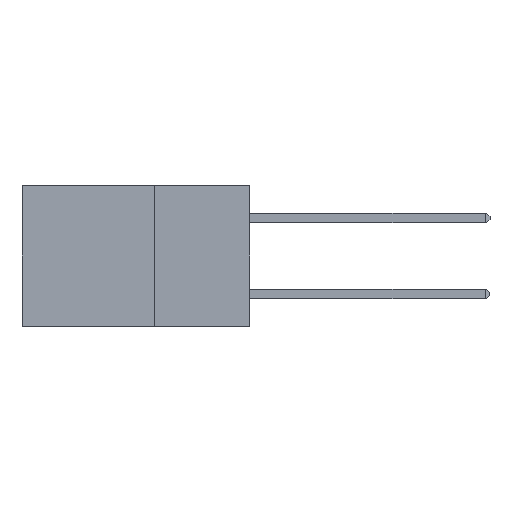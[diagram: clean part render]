
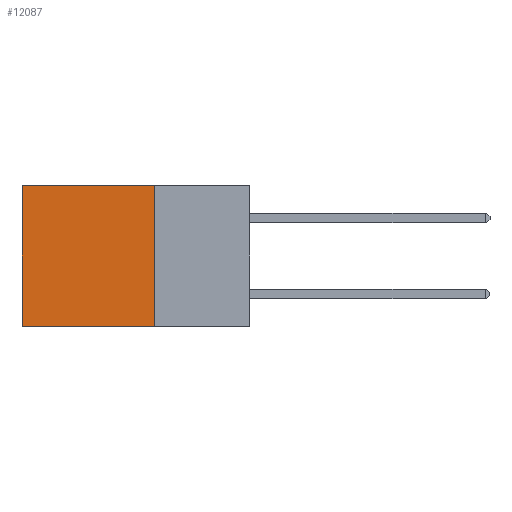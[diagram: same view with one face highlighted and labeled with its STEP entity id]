
A CAD part, left-side view. The second image highlights one B-rep face of the part: STEP entity #12087.
In plain terms, the highlighted planar face has unit normal (-1, 0, 0).
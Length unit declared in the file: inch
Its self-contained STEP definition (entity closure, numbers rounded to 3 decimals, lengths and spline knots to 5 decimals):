
#23 = CARTESIAN_POINT ( 'NONE',  ( 0.2875, 0.25, 0. ) ) ;
#40 = VECTOR ( 'NONE', #2135, 39.37008 ) ;
#397 = VECTOR ( 'NONE', #10074, 39.37008 ) ;
#904 = FACE_OUTER_BOUND ( 'NONE', #2620, .T. ) ;
#1497 = EDGE_CURVE ( 'NONE', #9863, #4979, #12409, .T. ) ;
#2125 = VERTEX_POINT ( 'NONE', #10823 ) ;
#2135 = DIRECTION ( 'NONE',  ( 0., 1., 0. ) ) ;
#2505 = CARTESIAN_POINT ( 'NONE',  ( 0.2875, 0.25, 0. ) ) ;
#2620 = EDGE_LOOP ( 'NONE', ( #8207, #11668, #6762, #9559 ) ) ;
#3856 = LINE ( 'NONE', #2505, #397 ) ;
#4747 = CARTESIAN_POINT ( 'NONE',  ( 0.2875, 0.25, 0. ) ) ;
#4979 = VERTEX_POINT ( 'NONE', #10751 ) ;
#5901 = CARTESIAN_POINT ( 'NONE',  ( 0.2875, 0.25, 0. ) ) ;
#6376 = EDGE_CURVE ( 'NONE', #4979, #8288, #9129, .T. ) ;
#6461 = DIRECTION ( 'NONE',  ( 0., 0., -1. ) ) ;
#6762 = ORIENTED_EDGE ( 'NONE', *, *, #15653, .F. ) ;
#7368 = CARTESIAN_POINT ( 'NONE',  ( 0.2875, 0.6, 0. ) ) ;
#8207 = ORIENTED_EDGE ( 'NONE', *, *, #6376, .T. ) ;
#8288 = VERTEX_POINT ( 'NONE', #11622 ) ;
#8626 = DIRECTION ( 'NONE',  ( 0., 0., -1. ) ) ;
#8936 = PLANE ( 'NONE',  #12317 ) ;
#9129 = LINE ( 'NONE', #7368, #12306 ) ;
#9242 = VECTOR ( 'NONE', #14485, 39.37008 ) ;
#9559 = ORIENTED_EDGE ( 'NONE', *, *, #1497, .T. ) ;
#9863 = VERTEX_POINT ( 'NONE', #5901 ) ;
#10074 = DIRECTION ( 'NONE',  ( 0., 0., -1. ) ) ;
#10751 = CARTESIAN_POINT ( 'NONE',  ( 0.2875, 0.6, 0. ) ) ;
#10823 = CARTESIAN_POINT ( 'NONE',  ( 0.2875, 0.25, -0.37 ) ) ;
#10930 = CARTESIAN_POINT ( 'NONE',  ( 0.2875, 0.25, -0.37 ) ) ;
#11622 = CARTESIAN_POINT ( 'NONE',  ( 0.2875, 0.6, -0.37 ) ) ;
#11668 = ORIENTED_EDGE ( 'NONE', *, *, #14819, .F. ) ;
#12087 = ADVANCED_FACE ( 'NONE', ( #904 ), #8936, .F. ) ;
#12306 = VECTOR ( 'NONE', #8626, 39.37008 ) ;
#12317 = AXIS2_PLACEMENT_3D ( 'NONE', #23, #13731, #6461 ) ;
#12409 = LINE ( 'NONE', #4747, #9242 ) ;
#12938 = LINE ( 'NONE', #10930, #40 ) ;
#13731 = DIRECTION ( 'NONE',  ( 1., 0., 0. ) ) ;
#14485 = DIRECTION ( 'NONE',  ( 0., 1., 0. ) ) ;
#14819 = EDGE_CURVE ( 'NONE', #2125, #8288, #12938, .T. ) ;
#15653 = EDGE_CURVE ( 'NONE', #9863, #2125, #3856, .T. ) ;
